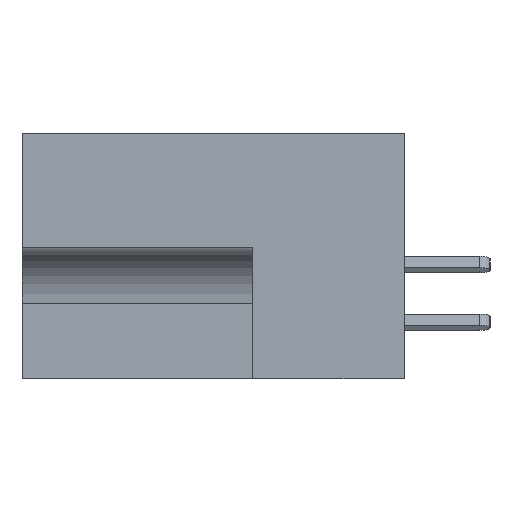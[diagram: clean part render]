
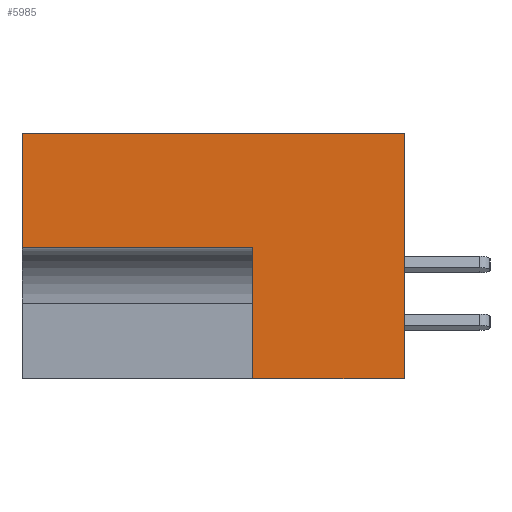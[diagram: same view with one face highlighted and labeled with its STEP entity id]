
A CAD part, left-side view. The second image highlights one B-rep face of the part: STEP entity #5985.
In plain terms, the highlighted planar face has unit normal (-1, 0, 0).
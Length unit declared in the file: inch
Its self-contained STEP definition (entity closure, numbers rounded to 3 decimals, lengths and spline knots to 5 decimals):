
#402 = PLANE ( 'NONE',  #15574 ) ;
#1098 = VERTEX_POINT ( 'NONE', #15360 ) ;
#1457 = DIRECTION ( 'NONE',  ( 0., 0., 1. ) ) ;
#2112 = EDGE_CURVE ( 'NONE', #21918, #15659, #4068, .T. ) ;
#2118 = DIRECTION ( 'NONE',  ( 0., 1., 0. ) ) ;
#2374 = CARTESIAN_POINT ( 'NONE',  ( 0., 0., 0. ) ) ;
#2649 = CARTESIAN_POINT ( 'NONE',  ( 0., 0.453, 0. ) ) ;
#4068 = LINE ( 'NONE', #9984, #7730 ) ;
#4095 = CARTESIAN_POINT ( 'NONE',  ( 0., 0.453, -0.531 ) ) ;
#4125 = ORIENTED_EDGE ( 'NONE', *, *, #6489, .F. ) ;
#4192 = CARTESIAN_POINT ( 'NONE',  ( 0., 0.453, 0. ) ) ;
#4640 = DIRECTION ( 'NONE',  ( 0., -1., 0. ) ) ;
#4672 = DIRECTION ( 'NONE',  ( 0., 0., 1. ) ) ;
#4706 = LINE ( 'NONE', #18363, #5534 ) ;
#5534 = VECTOR ( 'NONE', #2118, 39.37008 ) ;
#5623 = CARTESIAN_POINT ( 'NONE',  ( 0., 0., -0.531 ) ) ;
#5985 = ADVANCED_FACE ( 'NONE', ( #10254 ), #402, .F. ) ;
#6489 = EDGE_CURVE ( 'NONE', #1098, #18567, #15359, .T. ) ;
#7245 = VERTEX_POINT ( 'NONE', #5623 ) ;
#7730 = VECTOR ( 'NONE', #4672, 39.37008 ) ;
#8229 = ORIENTED_EDGE ( 'NONE', *, *, #9239, .T. ) ;
#8423 = DIRECTION ( 'NONE',  ( 0., -1., 0. ) ) ;
#9239 = EDGE_CURVE ( 'NONE', #21918, #7245, #14960, .T. ) ;
#9984 = CARTESIAN_POINT ( 'NONE',  ( 0., 0.328, -0.531 ) ) ;
#10083 = CARTESIAN_POINT ( 'NONE',  ( 0., 0.328, -0.531 ) ) ;
#10254 = FACE_OUTER_BOUND ( 'NONE', #15529, .T. ) ;
#10345 = EDGE_CURVE ( 'NONE', #15659, #16801, #4706, .T. ) ;
#11892 = EDGE_CURVE ( 'NONE', #16801, #1098, #21873, .T. ) ;
#12301 = ORIENTED_EDGE ( 'NONE', *, *, #2112, .F. ) ;
#13517 = CARTESIAN_POINT ( 'NONE',  ( 0., 0.328, -0.248 ) ) ;
#14069 = CARTESIAN_POINT ( 'NONE',  ( 0., 0., 0. ) ) ;
#14960 = LINE ( 'NONE', #4095, #22055 ) ;
#15359 = LINE ( 'NONE', #2649, #21334 ) ;
#15360 = CARTESIAN_POINT ( 'NONE',  ( 0., 0.828, 0. ) ) ;
#15529 = EDGE_LOOP ( 'NONE', ( #20736, #15869, #12301, #8229, #19090, #4125 ) ) ;
#15574 = AXIS2_PLACEMENT_3D ( 'NONE', #4192, #22255, #22101 ) ;
#15659 = VERTEX_POINT ( 'NONE', #13517 ) ;
#15662 = EDGE_CURVE ( 'NONE', #7245, #18567, #19427, .T. ) ;
#15869 = ORIENTED_EDGE ( 'NONE', *, *, #10345, .F. ) ;
#16719 = VECTOR ( 'NONE', #17009, 39.37008 ) ;
#16801 = VERTEX_POINT ( 'NONE', #23350 ) ;
#17009 = DIRECTION ( 'NONE',  ( 0., 0., 1. ) ) ;
#18363 = CARTESIAN_POINT ( 'NONE',  ( 0., 0.328, -0.248 ) ) ;
#18567 = VERTEX_POINT ( 'NONE', #2374 ) ;
#18855 = VECTOR ( 'NONE', #1457, 39.37008 ) ;
#19090 = ORIENTED_EDGE ( 'NONE', *, *, #15662, .T. ) ;
#19427 = LINE ( 'NONE', #14069, #18855 ) ;
#20583 = CARTESIAN_POINT ( 'NONE',  ( 0., 0.828, 0. ) ) ;
#20736 = ORIENTED_EDGE ( 'NONE', *, *, #11892, .F. ) ;
#21334 = VECTOR ( 'NONE', #8423, 39.37008 ) ;
#21873 = LINE ( 'NONE', #20583, #16719 ) ;
#21918 = VERTEX_POINT ( 'NONE', #10083 ) ;
#22055 = VECTOR ( 'NONE', #4640, 39.37008 ) ;
#22101 = DIRECTION ( 'NONE',  ( 0., 0., -1. ) ) ;
#22255 = DIRECTION ( 'NONE',  ( 1., 0., 0. ) ) ;
#23350 = CARTESIAN_POINT ( 'NONE',  ( 0., 0.828, -0.248 ) ) ;
